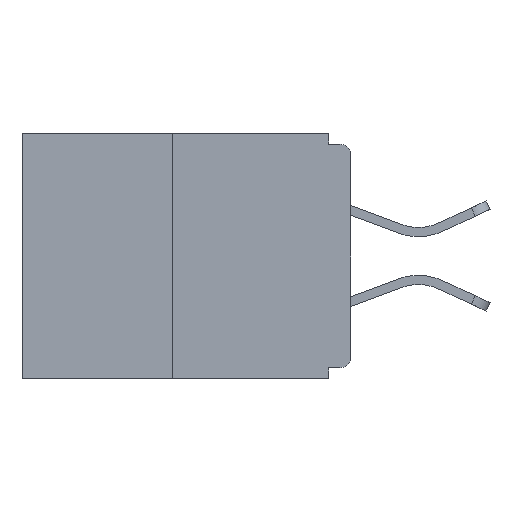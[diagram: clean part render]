
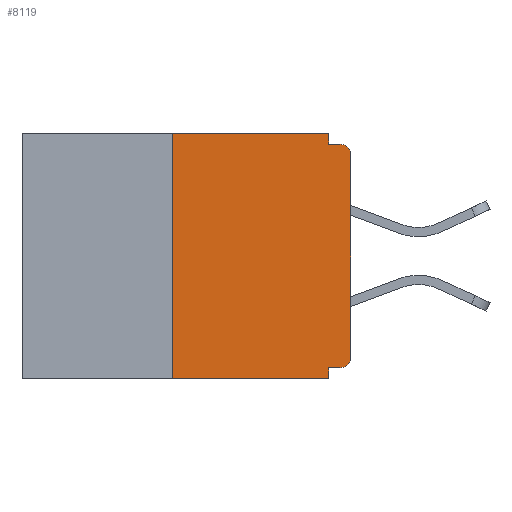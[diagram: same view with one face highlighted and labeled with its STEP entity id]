
A CAD part, left-side view. The second image highlights one B-rep face of the part: STEP entity #8119.
In plain terms, the highlighted planar face has unit normal (-1, 0, 0).
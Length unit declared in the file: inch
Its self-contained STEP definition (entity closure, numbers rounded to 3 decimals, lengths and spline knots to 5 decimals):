
#841 = DIRECTION ( 'NONE',  ( -1., 0., 0. ) ) ;
#1076 = VERTEX_POINT ( 'NONE', #8112 ) ;
#1123 = CARTESIAN_POINT ( 'NONE',  ( 0., 0.031, 0. ) ) ;
#1671 = DIRECTION ( 'NONE',  ( 0., 0., -1. ) ) ;
#2219 = LINE ( 'NONE', #2999, #14057 ) ;
#2229 = VECTOR ( 'NONE', #14894, 39.37008 ) ;
#2490 = LINE ( 'NONE', #7569, #4884 ) ;
#2731 = CIRCLE ( 'NONE', #12093, 0.015 ) ;
#2942 = EDGE_CURVE ( 'NONE', #1076, #5366, #10279, .T. ) ;
#2999 = CARTESIAN_POINT ( 'NONE',  ( 0., 0., 0. ) ) ;
#3091 = VERTEX_POINT ( 'NONE', #13521 ) ;
#3142 = DIRECTION ( 'NONE',  ( 1., 0., 0. ) ) ;
#3202 = LINE ( 'NONE', #13205, #2229 ) ;
#3678 = EDGE_CURVE ( 'NONE', #19567, #3091, #15802, .T. ) ;
#3963 = ORIENTED_EDGE ( 'NONE', *, *, #12754, .F. ) ;
#4163 = DIRECTION ( 'NONE',  ( 0., 0., -1. ) ) ;
#4474 = EDGE_CURVE ( 'NONE', #11663, #18991, #2731, .T. ) ;
#4692 = LINE ( 'NONE', #19939, #10258 ) ;
#4870 = CARTESIAN_POINT ( 'NONE',  ( 0., 0.015, -0.015 ) ) ;
#4884 = VECTOR ( 'NONE', #12259, 39.37008 ) ;
#5330 = VECTOR ( 'NONE', #5964, 39.37008 ) ;
#5335 = CARTESIAN_POINT ( 'NONE',  ( 0., 0.031, -0.015 ) ) ;
#5366 = VERTEX_POINT ( 'NONE', #7386 ) ;
#5470 = EDGE_CURVE ( 'NONE', #5366, #7519, #10642, .T. ) ;
#5964 = DIRECTION ( 'NONE',  ( 0., 0., -1. ) ) ;
#6086 = DIRECTION ( 'NONE',  ( 0., 0., 1. ) ) ;
#7071 = DIRECTION ( 'NONE',  ( 0., 0., -1. ) ) ;
#7386 = CARTESIAN_POINT ( 'NONE',  ( 0., 0.031, 0. ) ) ;
#7519 = VERTEX_POINT ( 'NONE', #5335 ) ;
#7532 = ORIENTED_EDGE ( 'NONE', *, *, #14097, .F. ) ;
#7569 = CARTESIAN_POINT ( 'NONE',  ( 0., 0., -0.015 ) ) ;
#7742 = LINE ( 'NONE', #15897, #15978 ) ;
#7982 = CARTESIAN_POINT ( 'NONE',  ( 0., 0.031, -0.328 ) ) ;
#8085 = EDGE_CURVE ( 'NONE', #17499, #12484, #4692, .T. ) ;
#8112 = CARTESIAN_POINT ( 'NONE',  ( 0., 0.25, 0. ) ) ;
#8119 = ADVANCED_FACE ( 'NONE', ( #19444 ), #18445, .F. ) ;
#8129 = AXIS2_PLACEMENT_3D ( 'NONE', #9345, #3142, #1671 ) ;
#9345 = CARTESIAN_POINT ( 'NONE',  ( 0., 0.46, 0. ) ) ;
#9789 = EDGE_LOOP ( 'NONE', ( #15998, #7532, #18062, #9813, #19323, #19800, #14282, #17190, #3963, #10021 ) ) ;
#9813 = ORIENTED_EDGE ( 'NONE', *, *, #15559, .F. ) ;
#9877 = EDGE_CURVE ( 'NONE', #19567, #10373, #7742, .T. ) ;
#10021 = ORIENTED_EDGE ( 'NONE', *, *, #5470, .F. ) ;
#10023 = CARTESIAN_POINT ( 'NONE',  ( 0., 0., -0.03 ) ) ;
#10258 = VECTOR ( 'NONE', #14822, 39.37008 ) ;
#10273 = EDGE_CURVE ( 'NONE', #3091, #11663, #2219, .T. ) ;
#10279 = LINE ( 'NONE', #19755, #11977 ) ;
#10373 = VERTEX_POINT ( 'NONE', #7982 ) ;
#10642 = LINE ( 'NONE', #1123, #5330 ) ;
#11663 = VERTEX_POINT ( 'NONE', #10023 ) ;
#11977 = VECTOR ( 'NONE', #16844, 39.37008 ) ;
#12093 = AXIS2_PLACEMENT_3D ( 'NONE', #19204, #841, #7071 ) ;
#12259 = DIRECTION ( 'NONE',  ( 0., -1., 0. ) ) ;
#12484 = VERTEX_POINT ( 'NONE', #15973 ) ;
#12754 = EDGE_CURVE ( 'NONE', #7519, #18991, #2490, .T. ) ;
#12990 = CARTESIAN_POINT ( 'NONE',  ( 0., 0.25, -0.343 ) ) ;
#13205 = CARTESIAN_POINT ( 'NONE',  ( 0., 0.25, 0. ) ) ;
#13521 = CARTESIAN_POINT ( 'NONE',  ( 0., 0., -0.313 ) ) ;
#13594 = DIRECTION ( 'NONE',  ( -1., 0., 0. ) ) ;
#14057 = VECTOR ( 'NONE', #6086, 39.37008 ) ;
#14097 = EDGE_CURVE ( 'NONE', #17499, #1076, #3202, .T. ) ;
#14215 = DIRECTION ( 'NONE',  ( 0., 1., 0. ) ) ;
#14282 = ORIENTED_EDGE ( 'NONE', *, *, #10273, .T. ) ;
#14822 = DIRECTION ( 'NONE',  ( 0., -1., 0. ) ) ;
#14894 = DIRECTION ( 'NONE',  ( 0., 0., 1. ) ) ;
#14947 = LINE ( 'NONE', #15087, #18561 ) ;
#15087 = CARTESIAN_POINT ( 'NONE',  ( 0., 0.031, -0.343 ) ) ;
#15559 = EDGE_CURVE ( 'NONE', #10373, #12484, #14947, .T. ) ;
#15802 = CIRCLE ( 'NONE', #18024, 0.015 ) ;
#15897 = CARTESIAN_POINT ( 'NONE',  ( 0., 0., -0.328 ) ) ;
#15973 = CARTESIAN_POINT ( 'NONE',  ( 0., 0.031, -0.343 ) ) ;
#15978 = VECTOR ( 'NONE', #14215, 39.37008 ) ;
#15998 = ORIENTED_EDGE ( 'NONE', *, *, #2942, .F. ) ;
#16619 = DIRECTION ( 'NONE',  ( 0., 0., -1. ) ) ;
#16844 = DIRECTION ( 'NONE',  ( 0., -1., 0. ) ) ;
#17190 = ORIENTED_EDGE ( 'NONE', *, *, #4474, .T. ) ;
#17499 = VERTEX_POINT ( 'NONE', #12990 ) ;
#18024 = AXIS2_PLACEMENT_3D ( 'NONE', #19742, #13594, #4163 ) ;
#18062 = ORIENTED_EDGE ( 'NONE', *, *, #8085, .T. ) ;
#18445 = PLANE ( 'NONE',  #8129 ) ;
#18561 = VECTOR ( 'NONE', #16619, 39.37008 ) ;
#18751 = CARTESIAN_POINT ( 'NONE',  ( 0., 0.015, -0.328 ) ) ;
#18991 = VERTEX_POINT ( 'NONE', #4870 ) ;
#19204 = CARTESIAN_POINT ( 'NONE',  ( 0., 0.015, -0.03 ) ) ;
#19323 = ORIENTED_EDGE ( 'NONE', *, *, #9877, .F. ) ;
#19444 = FACE_OUTER_BOUND ( 'NONE', #9789, .T. ) ;
#19567 = VERTEX_POINT ( 'NONE', #18751 ) ;
#19742 = CARTESIAN_POINT ( 'NONE',  ( 0., 0.015, -0.313 ) ) ;
#19755 = CARTESIAN_POINT ( 'NONE',  ( 0., 0.46, 0. ) ) ;
#19800 = ORIENTED_EDGE ( 'NONE', *, *, #3678, .T. ) ;
#19939 = CARTESIAN_POINT ( 'NONE',  ( 0., 0.46, -0.343 ) ) ;
